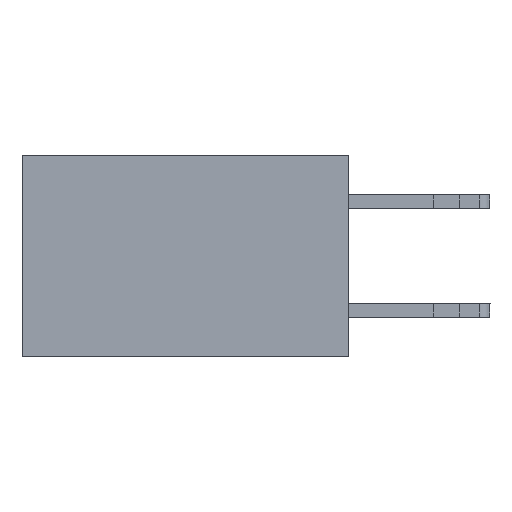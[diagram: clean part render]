
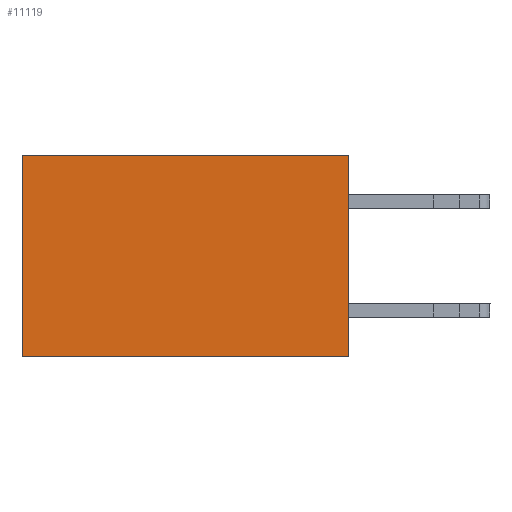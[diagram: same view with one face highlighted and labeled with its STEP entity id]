
A CAD part, left-side view. The second image highlights one B-rep face of the part: STEP entity #11119.
In plain terms, the highlighted planar face has unit normal (-1, 0, 0).
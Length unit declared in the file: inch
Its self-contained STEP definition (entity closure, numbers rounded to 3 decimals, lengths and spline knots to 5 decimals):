
#994 = CARTESIAN_POINT ( 'NONE',  ( 0.2615, 0., -0.37 ) ) ;
#2560 = VERTEX_POINT ( 'NONE', #2942 ) ;
#2942 = CARTESIAN_POINT ( 'NONE',  ( 0.2615, 0., 0. ) ) ;
#3426 = VECTOR ( 'NONE', #14932, 39.37008 ) ;
#3853 = VECTOR ( 'NONE', #6123, 39.37008 ) ;
#4144 = EDGE_CURVE ( 'NONE', #2560, #8129, #12765, .T. ) ;
#4604 = LINE ( 'NONE', #994, #9047 ) ;
#6123 = DIRECTION ( 'NONE',  ( 0., 0., -1. ) ) ;
#7858 = LINE ( 'NONE', #19951, #3426 ) ;
#8129 = VERTEX_POINT ( 'NONE', #15289 ) ;
#8309 = CARTESIAN_POINT ( 'NONE',  ( 0.2615, 0., -0.37 ) ) ;
#8476 = VERTEX_POINT ( 'NONE', #12682 ) ;
#9029 = ORIENTED_EDGE ( 'NONE', *, *, #4144, .F. ) ;
#9045 = ORIENTED_EDGE ( 'NONE', *, *, #17120, .F. ) ;
#9047 = VECTOR ( 'NONE', #12614, 39.37008 ) ;
#9922 = DIRECTION ( 'NONE',  ( 0., 0., -1. ) ) ;
#10166 = EDGE_LOOP ( 'NONE', ( #10393, #9045, #9029, #11168 ) ) ;
#10393 = ORIENTED_EDGE ( 'NONE', *, *, #17156, .T. ) ;
#11119 = ADVANCED_FACE ( 'NONE', ( #14524 ), #14746, .F. ) ;
#11168 = ORIENTED_EDGE ( 'NONE', *, *, #12664, .T. ) ;
#11911 = DIRECTION ( 'NONE',  ( 0., 0., -1. ) ) ;
#11937 = CARTESIAN_POINT ( 'NONE',  ( 0.2615, 0., -0.37 ) ) ;
#12614 = DIRECTION ( 'NONE',  ( 0., 1., 0. ) ) ;
#12664 = EDGE_CURVE ( 'NONE', #2560, #8476, #7858, .T. ) ;
#12682 = CARTESIAN_POINT ( 'NONE',  ( 0.2615, 0.6, 0. ) ) ;
#12765 = LINE ( 'NONE', #11937, #16573 ) ;
#13438 = CARTESIAN_POINT ( 'NONE',  ( 0.2615, 0.6, -0.37 ) ) ;
#14271 = CARTESIAN_POINT ( 'NONE',  ( 0.2615, 0.6, -0.37 ) ) ;
#14524 = FACE_OUTER_BOUND ( 'NONE', #10166, .T. ) ;
#14746 = PLANE ( 'NONE',  #14801 ) ;
#14801 = AXIS2_PLACEMENT_3D ( 'NONE', #8309, #19843, #9922 ) ;
#14932 = DIRECTION ( 'NONE',  ( 0., 1., 0. ) ) ;
#15289 = CARTESIAN_POINT ( 'NONE',  ( 0.2615, 0., -0.37 ) ) ;
#16573 = VECTOR ( 'NONE', #11911, 39.37008 ) ;
#16677 = LINE ( 'NONE', #14271, #3853 ) ;
#17120 = EDGE_CURVE ( 'NONE', #8129, #17456, #4604, .T. ) ;
#17156 = EDGE_CURVE ( 'NONE', #8476, #17456, #16677, .T. ) ;
#17456 = VERTEX_POINT ( 'NONE', #13438 ) ;
#19843 = DIRECTION ( 'NONE',  ( 1., 0., 0. ) ) ;
#19951 = CARTESIAN_POINT ( 'NONE',  ( 0.2615, 0., 0. ) ) ;
